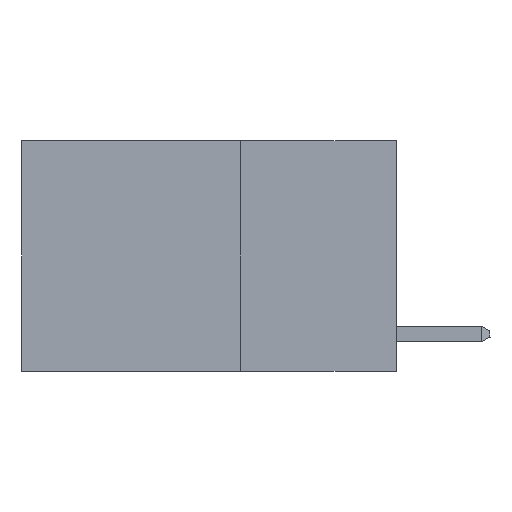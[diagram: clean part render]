
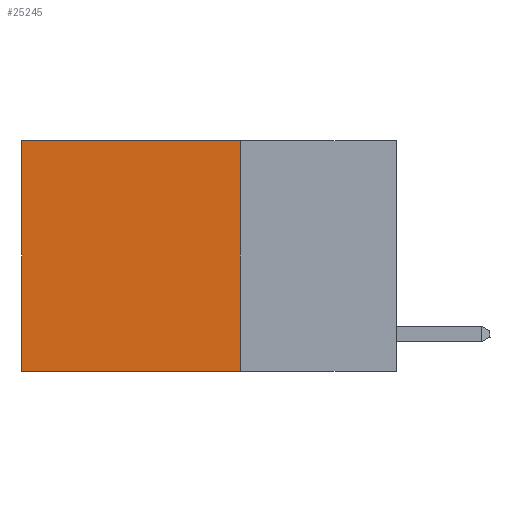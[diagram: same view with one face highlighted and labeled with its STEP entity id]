
A CAD part, left-side view. The second image highlights one B-rep face of the part: STEP entity #25245.
In plain terms, the highlighted planar face has unit normal (-1, 0, 0).
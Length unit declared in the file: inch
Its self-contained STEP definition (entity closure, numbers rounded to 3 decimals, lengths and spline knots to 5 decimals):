
#33 = VECTOR ( 'NONE', #18769, 39.37008 ) ;
#72 = FACE_OUTER_BOUND ( 'NONE', #9995, .T. ) ;
#115 = VECTOR ( 'NONE', #4748, 39.37008 ) ;
#583 = ORIENTED_EDGE ( 'NONE', *, *, #23347, .F. ) ;
#615 = VERTEX_POINT ( 'NONE', #24312 ) ;
#763 = LINE ( 'NONE', #5005, #33 ) ;
#2278 = LINE ( 'NONE', #4649, #115 ) ;
#2735 = CARTESIAN_POINT ( 'NONE',  ( 0.2625, 0.6, 0. ) ) ;
#3373 = DIRECTION ( 'NONE',  ( 0., 0., -1. ) ) ;
#3420 = VERTEX_POINT ( 'NONE', #10540 ) ;
#4649 = CARTESIAN_POINT ( 'NONE',  ( 0.2625, 0.25, -0.37 ) ) ;
#4748 = DIRECTION ( 'NONE',  ( 0., 1., 0. ) ) ;
#5005 = CARTESIAN_POINT ( 'NONE',  ( 0.2625, 0.25, 0. ) ) ;
#5075 = PLANE ( 'NONE',  #19782 ) ;
#7087 = DIRECTION ( 'NONE',  ( 0., 0., -1. ) ) ;
#7335 = DIRECTION ( 'NONE',  ( 0., 0., -1. ) ) ;
#9056 = ORIENTED_EDGE ( 'NONE', *, *, #11142, .T. ) ;
#9995 = EDGE_LOOP ( 'NONE', ( #9056, #27647, #583, #17330 ) ) ;
#10103 = VECTOR ( 'NONE', #3373, 39.37008 ) ;
#10540 = CARTESIAN_POINT ( 'NONE',  ( 0.2625, 0.6, -0.37 ) ) ;
#10824 = LINE ( 'NONE', #19427, #10103 ) ;
#10874 = VECTOR ( 'NONE', #7087, 39.37008 ) ;
#11142 = EDGE_CURVE ( 'NONE', #17894, #3420, #28352, .T. ) ;
#14064 = CARTESIAN_POINT ( 'NONE',  ( 0.2625, 0.6, 0. ) ) ;
#15274 = EDGE_CURVE ( 'NONE', #615, #3420, #2278, .T. ) ;
#16573 = EDGE_CURVE ( 'NONE', #26475, #17894, #763, .T. ) ;
#17330 = ORIENTED_EDGE ( 'NONE', *, *, #16573, .T. ) ;
#17894 = VERTEX_POINT ( 'NONE', #2735 ) ;
#18769 = DIRECTION ( 'NONE',  ( 0., 1., 0. ) ) ;
#18986 = CARTESIAN_POINT ( 'NONE',  ( 0.2625, 0.25, 0. ) ) ;
#19427 = CARTESIAN_POINT ( 'NONE',  ( 0.2625, 0.25, 0. ) ) ;
#19782 = AXIS2_PLACEMENT_3D ( 'NONE', #25502, #21113, #7335 ) ;
#21113 = DIRECTION ( 'NONE',  ( 1., 0., 0. ) ) ;
#23347 = EDGE_CURVE ( 'NONE', #26475, #615, #10824, .T. ) ;
#24312 = CARTESIAN_POINT ( 'NONE',  ( 0.2625, 0.25, -0.37 ) ) ;
#25245 = ADVANCED_FACE ( 'NONE', ( #72 ), #5075, .F. ) ;
#25502 = CARTESIAN_POINT ( 'NONE',  ( 0.2625, 0.25, 0. ) ) ;
#26475 = VERTEX_POINT ( 'NONE', #18986 ) ;
#27647 = ORIENTED_EDGE ( 'NONE', *, *, #15274, .F. ) ;
#28352 = LINE ( 'NONE', #14064, #10874 ) ;
